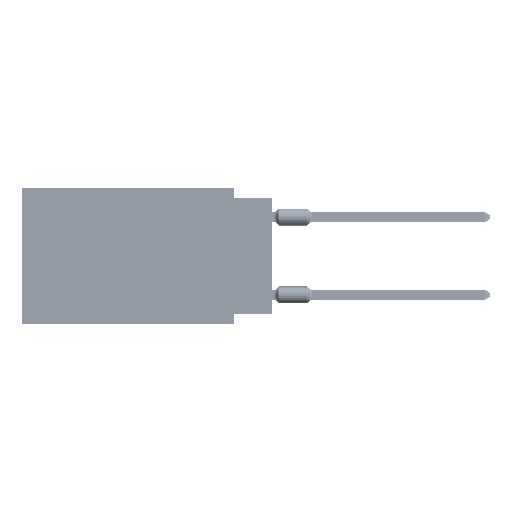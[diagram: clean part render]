
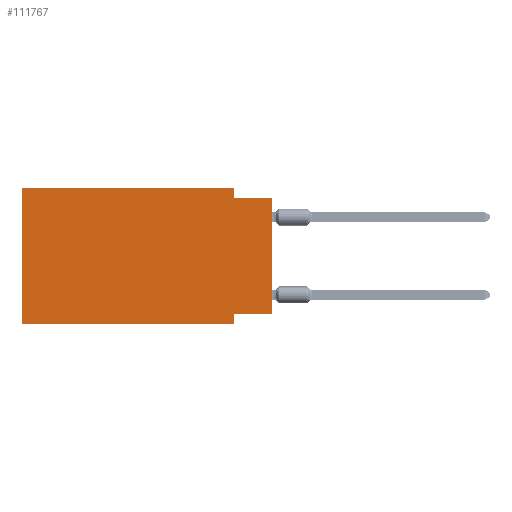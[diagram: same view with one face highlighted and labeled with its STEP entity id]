
A CAD part, left-side view. The second image highlights one B-rep face of the part: STEP entity #111767.
In plain terms, the highlighted planar face has unit normal (-1, 0, 0).
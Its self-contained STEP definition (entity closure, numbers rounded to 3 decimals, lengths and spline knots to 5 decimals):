
#3521 = CARTESIAN_POINT ( 'NONE',  ( 0., 0.645, -0.35 ) ) ;
#3756 = VECTOR ( 'NONE', #95939, 39.37008 ) ;
#5477 = VERTEX_POINT ( 'NONE', #71158 ) ;
#5756 = AXIS2_PLACEMENT_3D ( 'NONE', #97967, #80982, #79845 ) ;
#6843 = DIRECTION ( 'NONE',  ( 0., -1., 0. ) ) ;
#12630 = VERTEX_POINT ( 'NONE', #33232 ) ;
#12897 = CARTESIAN_POINT ( 'NONE',  ( 0., 0.1, -0.35 ) ) ;
#14158 = EDGE_CURVE ( 'NONE', #98678, #57370, #61765, .T. ) ;
#14806 = CARTESIAN_POINT ( 'NONE',  ( 0., 0.1, 0. ) ) ;
#15300 = VECTOR ( 'NONE', #109400, 39.37008 ) ;
#15588 = VERTEX_POINT ( 'NONE', #29009 ) ;
#19486 = DIRECTION ( 'NONE',  ( 0., 1., 0. ) ) ;
#26163 = DIRECTION ( 'NONE',  ( 0., -1., 0. ) ) ;
#29009 = CARTESIAN_POINT ( 'NONE',  ( 0., 0.1, -0.325 ) ) ;
#30639 = VECTOR ( 'NONE', #41619, 39.37008 ) ;
#31772 = CARTESIAN_POINT ( 'NONE',  ( 0., 0.1, -0.025 ) ) ;
#33130 = EDGE_CURVE ( 'NONE', #15588, #83285, #73700, .T. ) ;
#33232 = CARTESIAN_POINT ( 'NONE',  ( 0., 0., -0.025 ) ) ;
#33768 = EDGE_CURVE ( 'NONE', #103497, #12630, #78756, .T. ) ;
#33805 = ORIENTED_EDGE ( 'NONE', *, *, #110718, .T. ) ;
#34281 = PLANE ( 'NONE',  #5756 ) ;
#35927 = VECTOR ( 'NONE', #26163, 39.37008 ) ;
#37046 = LINE ( 'NONE', #91380, #58143 ) ;
#40236 = CARTESIAN_POINT ( 'NONE',  ( 0., 0.645, -0.35 ) ) ;
#40833 = ORIENTED_EDGE ( 'NONE', *, *, #45198, .F. ) ;
#41619 = DIRECTION ( 'NONE',  ( 0., 0., 1. ) ) ;
#43094 = ORIENTED_EDGE ( 'NONE', *, *, #85791, .F. ) ;
#44034 = ORIENTED_EDGE ( 'NONE', *, *, #33130, .F. ) ;
#44675 = CARTESIAN_POINT ( 'NONE',  ( 0., 0.1, -0.35 ) ) ;
#45198 = EDGE_CURVE ( 'NONE', #5477, #15588, #37046, .T. ) ;
#54193 = EDGE_CURVE ( 'NONE', #82141, #83285, #58324, .T. ) ;
#56163 = CARTESIAN_POINT ( 'NONE',  ( 0., 0.1, 0. ) ) ;
#57370 = VERTEX_POINT ( 'NONE', #56163 ) ;
#58143 = VECTOR ( 'NONE', #19486, 39.37008 ) ;
#58324 = LINE ( 'NONE', #40236, #59156 ) ;
#59156 = VECTOR ( 'NONE', #75857, 39.37008 ) ;
#60282 = CARTESIAN_POINT ( 'NONE',  ( 0., 0., 0. ) ) ;
#61765 = LINE ( 'NONE', #76986, #86272 ) ;
#64089 = EDGE_CURVE ( 'NONE', #57370, #103497, #91438, .T. ) ;
#65588 = VECTOR ( 'NONE', #84393, 39.37008 ) ;
#66748 = CARTESIAN_POINT ( 'NONE',  ( 0., 0.645, 0. ) ) ;
#71158 = CARTESIAN_POINT ( 'NONE',  ( 0., 0., -0.325 ) ) ;
#73700 = LINE ( 'NONE', #12897, #15300 ) ;
#75857 = DIRECTION ( 'NONE',  ( 0., -1., 0. ) ) ;
#76760 = EDGE_LOOP ( 'NONE', ( #33805, #106739, #87348, #103873, #43094, #104898, #44034, #40833 ) ) ;
#76986 = CARTESIAN_POINT ( 'NONE',  ( 0., 0.645, 0. ) ) ;
#78756 = LINE ( 'NONE', #106243, #35927 ) ;
#79845 = DIRECTION ( 'NONE',  ( 0., 0., -1. ) ) ;
#80982 = DIRECTION ( 'NONE',  ( 1., 0., 0. ) ) ;
#82141 = VERTEX_POINT ( 'NONE', #3521 ) ;
#83285 = VERTEX_POINT ( 'NONE', #44675 ) ;
#84393 = DIRECTION ( 'NONE',  ( 0., 0., -1. ) ) ;
#84867 = LINE ( 'NONE', #66748, #30639 ) ;
#85791 = EDGE_CURVE ( 'NONE', #82141, #98678, #84867, .T. ) ;
#86272 = VECTOR ( 'NONE', #6843, 39.37008 ) ;
#87348 = ORIENTED_EDGE ( 'NONE', *, *, #64089, .F. ) ;
#91380 = CARTESIAN_POINT ( 'NONE',  ( 0., 0., -0.325 ) ) ;
#91438 = LINE ( 'NONE', #14806, #65588 ) ;
#95939 = DIRECTION ( 'NONE',  ( 0., 0., 1. ) ) ;
#96248 = FACE_OUTER_BOUND ( 'NONE', #76760, .T. ) ;
#97967 = CARTESIAN_POINT ( 'NONE',  ( 0., 0.645, 0. ) ) ;
#98396 = CARTESIAN_POINT ( 'NONE',  ( 0., 0.645, 0. ) ) ;
#98678 = VERTEX_POINT ( 'NONE', #98396 ) ;
#103497 = VERTEX_POINT ( 'NONE', #31772 ) ;
#103873 = ORIENTED_EDGE ( 'NONE', *, *, #14158, .F. ) ;
#104898 = ORIENTED_EDGE ( 'NONE', *, *, #54193, .T. ) ;
#106243 = CARTESIAN_POINT ( 'NONE',  ( 0., 0., -0.025 ) ) ;
#106739 = ORIENTED_EDGE ( 'NONE', *, *, #33768, .F. ) ;
#109400 = DIRECTION ( 'NONE',  ( 0., 0., -1. ) ) ;
#110718 = EDGE_CURVE ( 'NONE', #5477, #12630, #113499, .T. ) ;
#111767 = ADVANCED_FACE ( 'NONE', ( #96248 ), #34281, .F. ) ;
#113499 = LINE ( 'NONE', #60282, #3756 ) ;
